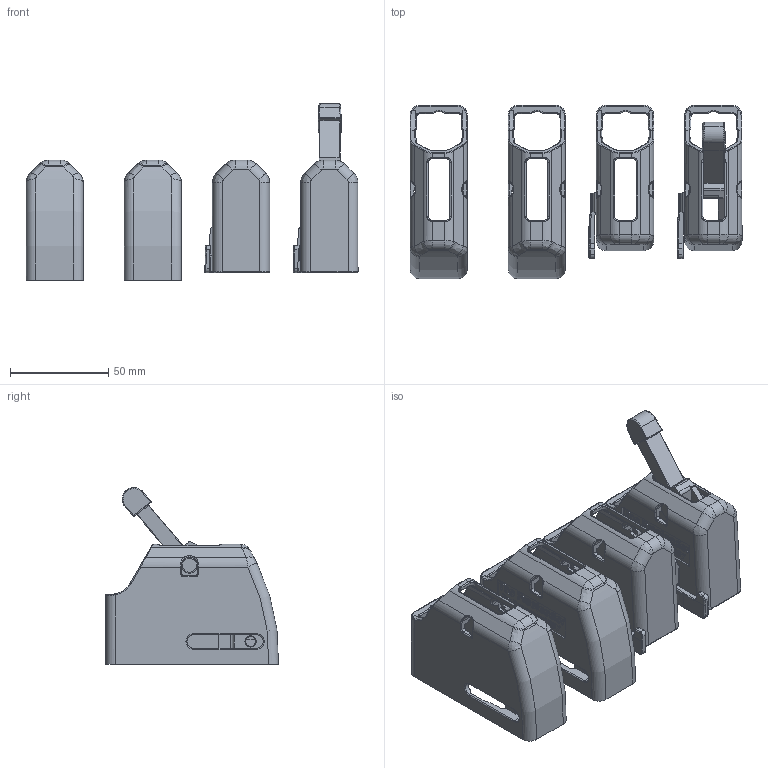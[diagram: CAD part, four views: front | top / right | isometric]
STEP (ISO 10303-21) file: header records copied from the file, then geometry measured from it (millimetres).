
FILE_DESCRIPTION(/* description */ (''),/* implementation_level */ '2;1');
FILE_NAME(/* name */ 'TheFreeloader-ar15-release-all-final.step',/* time_stamp */ '2021-09-20T14:53:25-07:00',/* author */ (''),/* organization */ (''),/* preprocessor_version */ 'ST-DEVELOPER v18.1',/* originating_system */ 'Autodesk Translation Framework v10.10.0.1391',/* authorisation */ '');
FILE_SCHEMA (('AUTOMOTIVE_DESIGN { 1 0 10303 214 3 1 1 }'));
Products named in the file (1): TheFreeloader-ar15-release-sanatized
Bounding box: 169.22 x 88.21 x 90.19 mm (x, y, z)
Volume: 157231.8 mm3; surface area: 93680.8 mm2
Topology: 5 solids, 5 shells, 5709 faces, 15392 edges, 10003 vertices
Faces by surface type: bspline 3221, plane 1682, cylinder 568, torus 222, cone 12, sphere 4
Full cylindrical faces by diameter (mm): 5.182 x2, 7.925 x2, 8.12 x2
Entity records: 203341 total; most frequent: CARTESIAN_POINT 84683, ORIENTED_EDGE 30770, DIRECTION 16704, EDGE_CURVE 15385, VERTEX_POINT 10003, LINE 7204, VECTOR 7204, EDGE_LOOP 6066
